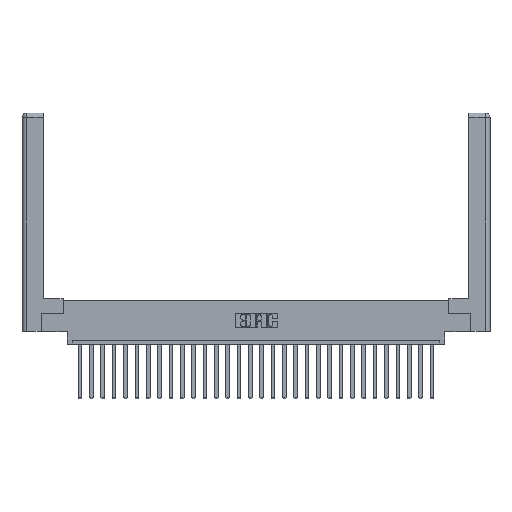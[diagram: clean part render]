
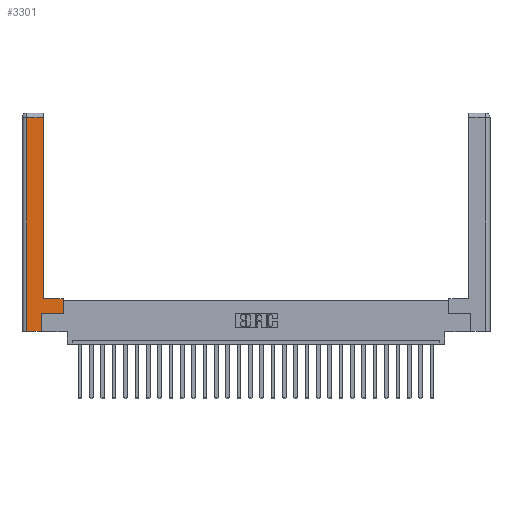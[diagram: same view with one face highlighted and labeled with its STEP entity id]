
A CAD part, top view. The second image highlights one B-rep face of the part: STEP entity #3301.
In plain terms, the highlighted planar face has unit normal (0, 0, 1).
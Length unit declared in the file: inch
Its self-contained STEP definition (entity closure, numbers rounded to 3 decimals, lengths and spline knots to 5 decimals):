
#420 = LINE ( 'NONE', #16688, #10473 ) ;
#1153 = LINE ( 'NONE', #10218, #25936 ) ;
#1640 = VECTOR ( 'NONE', #11642, 39.37008 ) ;
#1676 = EDGE_CURVE ( 'NONE', #19534, #4125, #23622, .T. ) ;
#1935 = DIRECTION ( 'NONE',  ( 0., 1., 0. ) ) ;
#2128 = CARTESIAN_POINT ( 'NONE',  ( 0.295, 2.94, 0. ) ) ;
#2176 = EDGE_LOOP ( 'NONE', ( #7966, #18092, #18921, #12709, #10355, #13249, #10856, #18333 ) ) ;
#3301 = ADVANCED_FACE ( 'NONE', ( #7811 ), #4137, .F. ) ;
#3326 = LINE ( 'NONE', #8103, #26724 ) ;
#3808 = DIRECTION ( 'NONE',  ( -1., 0., 0. ) ) ;
#4125 = VERTEX_POINT ( 'NONE', #21746 ) ;
#4137 = PLANE ( 'NONE',  #5326 ) ;
#4439 = CARTESIAN_POINT ( 'NONE',  ( 0.265, 0., 0. ) ) ;
#4732 = DIRECTION ( 'NONE',  ( 1., 0., 0. ) ) ;
#5326 = AXIS2_PLACEMENT_3D ( 'NONE', #23298, #26886, #3808 ) ;
#5391 = VERTEX_POINT ( 'NONE', #10526 ) ;
#6610 = VECTOR ( 'NONE', #19208, 39.37008 ) ;
#7811 = FACE_OUTER_BOUND ( 'NONE', #2176, .T. ) ;
#7907 = VECTOR ( 'NONE', #20953, 39.37008 ) ;
#7966 = ORIENTED_EDGE ( 'NONE', *, *, #12973, .T. ) ;
#8103 = CARTESIAN_POINT ( 'NONE',  ( 0.0615, 0., 0. ) ) ;
#8193 = LINE ( 'NONE', #21605, #18235 ) ;
#8873 = EDGE_CURVE ( 'NONE', #14254, #19729, #3326, .T. ) ;
#9640 = CARTESIAN_POINT ( 'NONE',  ( 0.265, 0.245, 0. ) ) ;
#10124 = CARTESIAN_POINT ( 'NONE',  ( 0.0615, 2.94, 0. ) ) ;
#10218 = CARTESIAN_POINT ( 'NONE',  ( 0.565, 0.45, 0. ) ) ;
#10355 = ORIENTED_EDGE ( 'NONE', *, *, #24972, .T. ) ;
#10473 = VECTOR ( 'NONE', #1935, 39.37008 ) ;
#10526 = CARTESIAN_POINT ( 'NONE',  ( 0.295, 0.45, 0. ) ) ;
#10544 = EDGE_CURVE ( 'NONE', #26593, #14254, #17991, .T. ) ;
#10856 = ORIENTED_EDGE ( 'NONE', *, *, #23177, .T. ) ;
#11642 = DIRECTION ( 'NONE',  ( 0., 1., 0. ) ) ;
#11830 = CARTESIAN_POINT ( 'NONE',  ( 0.0615, 2.94, 0. ) ) ;
#12709 = ORIENTED_EDGE ( 'NONE', *, *, #18644, .T. ) ;
#12973 = EDGE_CURVE ( 'NONE', #5391, #26593, #18043, .T. ) ;
#13249 = ORIENTED_EDGE ( 'NONE', *, *, #1676, .T. ) ;
#14254 = VERTEX_POINT ( 'NONE', #11830 ) ;
#14448 = VECTOR ( 'NONE', #4732, 39.37008 ) ;
#14780 = LINE ( 'NONE', #4439, #14448 ) ;
#16355 = DIRECTION ( 'NONE',  ( 0., 1., 0. ) ) ;
#16688 = CARTESIAN_POINT ( 'NONE',  ( 0.265, 0.245, 0. ) ) ;
#17174 = EDGE_CURVE ( 'NONE', #23694, #5391, #8193, .T. ) ;
#17751 = VERTEX_POINT ( 'NONE', #18722 ) ;
#17991 = LINE ( 'NONE', #10124, #6610 ) ;
#18043 = LINE ( 'NONE', #19648, #1640 ) ;
#18092 = ORIENTED_EDGE ( 'NONE', *, *, #10544, .T. ) ;
#18235 = VECTOR ( 'NONE', #24146, 39.37008 ) ;
#18333 = ORIENTED_EDGE ( 'NONE', *, *, #17174, .T. ) ;
#18565 = DIRECTION ( 'NONE',  ( 0., -1., 0. ) ) ;
#18644 = EDGE_CURVE ( 'NONE', #19729, #17751, #14780, .T. ) ;
#18722 = CARTESIAN_POINT ( 'NONE',  ( 0.265, 0., 0. ) ) ;
#18921 = ORIENTED_EDGE ( 'NONE', *, *, #8873, .T. ) ;
#19208 = DIRECTION ( 'NONE',  ( -1., 0., 0. ) ) ;
#19534 = VERTEX_POINT ( 'NONE', #9640 ) ;
#19648 = CARTESIAN_POINT ( 'NONE',  ( 0.295, 3., 0. ) ) ;
#19729 = VERTEX_POINT ( 'NONE', #21419 ) ;
#20076 = CARTESIAN_POINT ( 'NONE',  ( 0.565, 0.45, 0. ) ) ;
#20953 = DIRECTION ( 'NONE',  ( 1., 0., 0. ) ) ;
#21419 = CARTESIAN_POINT ( 'NONE',  ( 0.0615, 0., 0. ) ) ;
#21605 = CARTESIAN_POINT ( 'NONE',  ( 0.295, 0.45, 0. ) ) ;
#21746 = CARTESIAN_POINT ( 'NONE',  ( 0.565, 0.245, 0. ) ) ;
#23177 = EDGE_CURVE ( 'NONE', #4125, #23694, #1153, .T. ) ;
#23298 = CARTESIAN_POINT ( 'NONE',  ( 0., 0., 0. ) ) ;
#23622 = LINE ( 'NONE', #24882, #7907 ) ;
#23694 = VERTEX_POINT ( 'NONE', #20076 ) ;
#24146 = DIRECTION ( 'NONE',  ( -1., 0., 0. ) ) ;
#24882 = CARTESIAN_POINT ( 'NONE',  ( 0.565, 0.245, 0. ) ) ;
#24972 = EDGE_CURVE ( 'NONE', #17751, #19534, #420, .T. ) ;
#25936 = VECTOR ( 'NONE', #16355, 39.37008 ) ;
#26593 = VERTEX_POINT ( 'NONE', #2128 ) ;
#26724 = VECTOR ( 'NONE', #18565, 39.37008 ) ;
#26886 = DIRECTION ( 'NONE',  ( 0., 0., -1. ) ) ;
